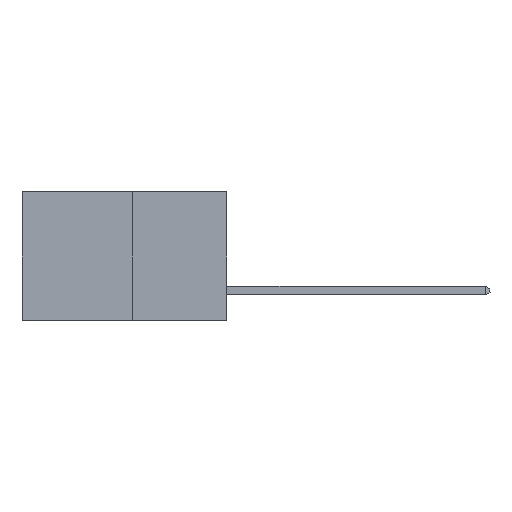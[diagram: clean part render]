
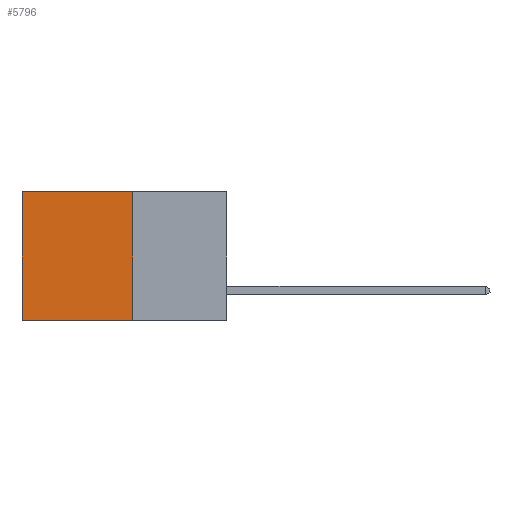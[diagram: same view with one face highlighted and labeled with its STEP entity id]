
A CAD part, left-side view. The second image highlights one B-rep face of the part: STEP entity #5796.
In plain terms, the highlighted planar face has unit normal (-1, 0, 0).
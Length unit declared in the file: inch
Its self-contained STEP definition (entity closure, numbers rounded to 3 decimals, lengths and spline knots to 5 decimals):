
#11 = VERTEX_POINT ( 'NONE', #5525 ) ;
#785 = EDGE_CURVE ( 'NONE', #3310, #4703, #8759, .T. ) ;
#1012 = PLANE ( 'NONE',  #8596 ) ;
#1041 = CARTESIAN_POINT ( 'NONE',  ( 0.277, 0.27, 0. ) ) ;
#1101 = LINE ( 'NONE', #7244, #4998 ) ;
#1188 = LINE ( 'NONE', #9053, #8590 ) ;
#1297 = ORIENTED_EDGE ( 'NONE', *, *, #2294, .T. ) ;
#1624 = DIRECTION ( 'NONE',  ( 0., 1., 0. ) ) ;
#2294 = EDGE_CURVE ( 'NONE', #4703, #11, #1101, .T. ) ;
#2427 = CARTESIAN_POINT ( 'NONE',  ( 0.277, 0.27, -0.37 ) ) ;
#2486 = DIRECTION ( 'NONE',  ( 0., 0., -1. ) ) ;
#2542 = DIRECTION ( 'NONE',  ( 0., 0., -1. ) ) ;
#2705 = VECTOR ( 'NONE', #9040, 39.37008 ) ;
#3310 = VERTEX_POINT ( 'NONE', #1041 ) ;
#3937 = ORIENTED_EDGE ( 'NONE', *, *, #8943, .F. ) ;
#4249 = EDGE_LOOP ( 'NONE', ( #1297, #3937, #6953, #4335 ) ) ;
#4335 = ORIENTED_EDGE ( 'NONE', *, *, #785, .T. ) ;
#4551 = VECTOR ( 'NONE', #1624, 39.37008 ) ;
#4703 = VERTEX_POINT ( 'NONE', #5073 ) ;
#4705 = DIRECTION ( 'NONE',  ( 1., 0., 0. ) ) ;
#4998 = VECTOR ( 'NONE', #5312, 39.37008 ) ;
#5073 = CARTESIAN_POINT ( 'NONE',  ( 0.277, 0.59, 0. ) ) ;
#5312 = DIRECTION ( 'NONE',  ( 0., 0., -1. ) ) ;
#5525 = CARTESIAN_POINT ( 'NONE',  ( 0.277, 0.59, -0.37 ) ) ;
#5796 = ADVANCED_FACE ( 'NONE', ( #7378 ), #1012, .F. ) ;
#6208 = CARTESIAN_POINT ( 'NONE',  ( 0.277, 0.27, -0.37 ) ) ;
#6472 = VERTEX_POINT ( 'NONE', #6208 ) ;
#6695 = EDGE_CURVE ( 'NONE', #3310, #6472, #1188, .T. ) ;
#6953 = ORIENTED_EDGE ( 'NONE', *, *, #6695, .F. ) ;
#7244 = CARTESIAN_POINT ( 'NONE',  ( 0.277, 0.59, -0.37 ) ) ;
#7378 = FACE_OUTER_BOUND ( 'NONE', #4249, .T. ) ;
#7417 = CARTESIAN_POINT ( 'NONE',  ( 0.277, 0.27, -0.37 ) ) ;
#8590 = VECTOR ( 'NONE', #2542, 39.37008 ) ;
#8596 = AXIS2_PLACEMENT_3D ( 'NONE', #7417, #4705, #2486 ) ;
#8756 = LINE ( 'NONE', #2427, #4551 ) ;
#8759 = LINE ( 'NONE', #9023, #2705 ) ;
#8943 = EDGE_CURVE ( 'NONE', #6472, #11, #8756, .T. ) ;
#9023 = CARTESIAN_POINT ( 'NONE',  ( 0.277, 0.27, 0. ) ) ;
#9040 = DIRECTION ( 'NONE',  ( 0., 1., 0. ) ) ;
#9053 = CARTESIAN_POINT ( 'NONE',  ( 0.277, 0.27, -0.37 ) ) ;
